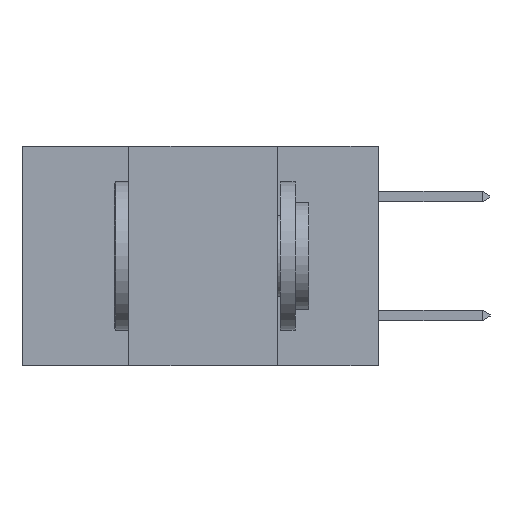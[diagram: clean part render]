
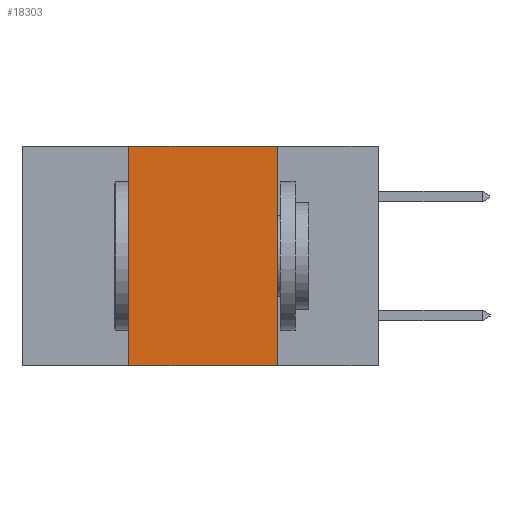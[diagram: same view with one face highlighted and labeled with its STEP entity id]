
A CAD part, left-side view. The second image highlights one B-rep face of the part: STEP entity #18303.
In plain terms, the highlighted planar face has unit normal (-1, 0, 0).
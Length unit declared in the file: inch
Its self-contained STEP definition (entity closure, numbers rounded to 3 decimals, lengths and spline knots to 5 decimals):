
#202 = VERTEX_POINT ( 'NONE', #14281 ) ;
#532 = DIRECTION ( 'NONE',  ( 0., -1., 0. ) ) ;
#624 = VECTOR ( 'NONE', #532, 39.37008 ) ;
#1180 = DIRECTION ( 'NONE',  ( 0., 0., -1. ) ) ;
#1441 = DIRECTION ( 'NONE',  ( 0., -1., 0. ) ) ;
#1468 = CARTESIAN_POINT ( 'NONE',  ( 0., 0.42, 0. ) ) ;
#1972 = VERTEX_POINT ( 'NONE', #2778 ) ;
#2778 = CARTESIAN_POINT ( 'NONE',  ( 0., 0.42, -0.37 ) ) ;
#4301 = ORIENTED_EDGE ( 'NONE', *, *, #22267, .F. ) ;
#4354 = CARTESIAN_POINT ( 'NONE',  ( 0., 0.6, 0. ) ) ;
#4378 = ORIENTED_EDGE ( 'NONE', *, *, #16581, .F. ) ;
#4758 = LINE ( 'NONE', #9980, #14607 ) ;
#5370 = ORIENTED_EDGE ( 'NONE', *, *, #7870, .T. ) ;
#6475 = DIRECTION ( 'NONE',  ( 0., 0., -1. ) ) ;
#6594 = ORIENTED_EDGE ( 'NONE', *, *, #25680, .F. ) ;
#6912 = LINE ( 'NONE', #15251, #624 ) ;
#7870 = EDGE_CURVE ( 'NONE', #1972, #12548, #4758, .T. ) ;
#9980 = CARTESIAN_POINT ( 'NONE',  ( 0., 0.6, -0.37 ) ) ;
#10080 = FACE_OUTER_BOUND ( 'NONE', #22972, .T. ) ;
#10372 = AXIS2_PLACEMENT_3D ( 'NONE', #4354, #18947, #6475 ) ;
#10385 = LINE ( 'NONE', #26295, #20719 ) ;
#12548 = VERTEX_POINT ( 'NONE', #14989 ) ;
#13792 = CARTESIAN_POINT ( 'NONE',  ( 0., 0.17, -0.37 ) ) ;
#14027 = LINE ( 'NONE', #13792, #25584 ) ;
#14281 = CARTESIAN_POINT ( 'NONE',  ( 0., 0.17, 0. ) ) ;
#14607 = VECTOR ( 'NONE', #1441, 39.37008 ) ;
#14806 = PLANE ( 'NONE',  #10372 ) ;
#14989 = CARTESIAN_POINT ( 'NONE',  ( 0., 0.17, -0.37 ) ) ;
#15251 = CARTESIAN_POINT ( 'NONE',  ( 0., 0.6, 0. ) ) ;
#16581 = EDGE_CURVE ( 'NONE', #202, #12548, #14027, .T. ) ;
#18158 = DIRECTION ( 'NONE',  ( 0., 0., 1. ) ) ;
#18303 = ADVANCED_FACE ( 'NONE', ( #10080 ), #14806, .F. ) ;
#18947 = DIRECTION ( 'NONE',  ( 1., 0., 0. ) ) ;
#20719 = VECTOR ( 'NONE', #18158, 39.37008 ) ;
#22267 = EDGE_CURVE ( 'NONE', #1972, #24947, #10385, .T. ) ;
#22972 = EDGE_LOOP ( 'NONE', ( #4378, #6594, #4301, #5370 ) ) ;
#24947 = VERTEX_POINT ( 'NONE', #1468 ) ;
#25584 = VECTOR ( 'NONE', #1180, 39.37008 ) ;
#25680 = EDGE_CURVE ( 'NONE', #24947, #202, #6912, .T. ) ;
#26295 = CARTESIAN_POINT ( 'NONE',  ( 0., 0.42, -0.37 ) ) ;
